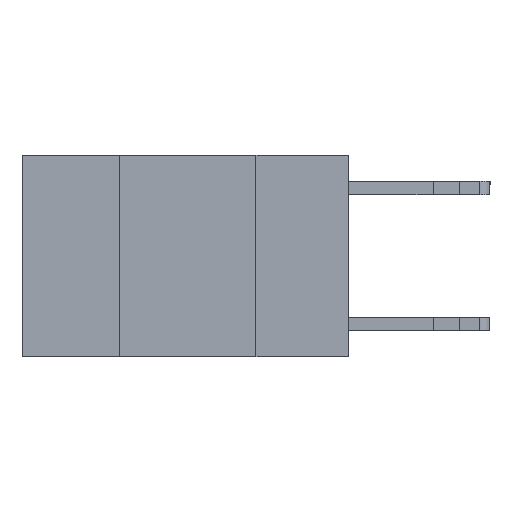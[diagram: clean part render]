
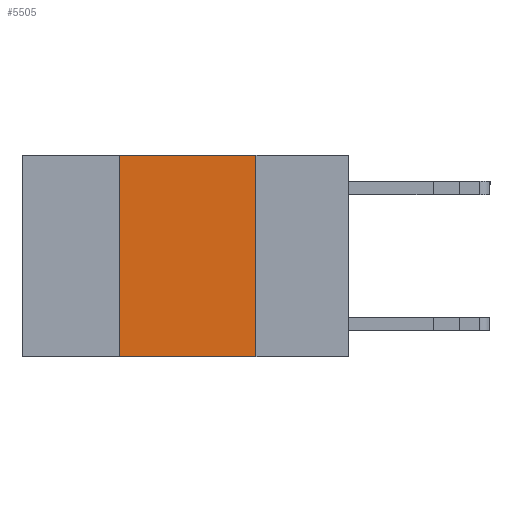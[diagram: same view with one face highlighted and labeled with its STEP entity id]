
A CAD part, left-side view. The second image highlights one B-rep face of the part: STEP entity #5505.
In plain terms, the highlighted planar face has unit normal (-1, 0, 0).
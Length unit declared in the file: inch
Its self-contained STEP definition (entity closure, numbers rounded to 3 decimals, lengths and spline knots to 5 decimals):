
#388 = LINE ( 'NONE', #5888, #15726 ) ;
#2039 = ORIENTED_EDGE ( 'NONE', *, *, #4509, .F. ) ;
#2370 = CARTESIAN_POINT ( 'NONE',  ( 0., 0.42, 0. ) ) ;
#3169 = DIRECTION ( 'NONE',  ( 0., -1., 0. ) ) ;
#3200 = CARTESIAN_POINT ( 'NONE',  ( 0., 0.17, -0.37 ) ) ;
#3448 = VERTEX_POINT ( 'NONE', #3200 ) ;
#3817 = DIRECTION ( 'NONE',  ( 0., 0., 1. ) ) ;
#4509 = EDGE_CURVE ( 'NONE', #7528, #14294, #9182, .T. ) ;
#5053 = ORIENTED_EDGE ( 'NONE', *, *, #5731, .T. ) ;
#5300 = DIRECTION ( 'NONE',  ( 0., 0., -1. ) ) ;
#5437 = VECTOR ( 'NONE', #7919, 39.37008 ) ;
#5505 = ADVANCED_FACE ( 'NONE', ( #9479 ), #9311, .F. ) ;
#5697 = VECTOR ( 'NONE', #11566, 39.37008 ) ;
#5731 = EDGE_CURVE ( 'NONE', #14830, #3448, #388, .T. ) ;
#5888 = CARTESIAN_POINT ( 'NONE',  ( 0., 0.6, -0.37 ) ) ;
#7187 = AXIS2_PLACEMENT_3D ( 'NONE', #17569, #13532, #5300 ) ;
#7528 = VERTEX_POINT ( 'NONE', #15100 ) ;
#7919 = DIRECTION ( 'NONE',  ( 0., 0., -1. ) ) ;
#8011 = CARTESIAN_POINT ( 'NONE',  ( 0., 0.42, -0.37 ) ) ;
#9182 = LINE ( 'NONE', #14190, #5697 ) ;
#9247 = LINE ( 'NONE', #9504, #5437 ) ;
#9311 = PLANE ( 'NONE',  #7187 ) ;
#9479 = FACE_OUTER_BOUND ( 'NONE', #15488, .T. ) ;
#9504 = CARTESIAN_POINT ( 'NONE',  ( 0., 0.17, 0. ) ) ;
#10403 = ORIENTED_EDGE ( 'NONE', *, *, #16967, .F. ) ;
#11566 = DIRECTION ( 'NONE',  ( 0., -1., 0. ) ) ;
#13428 = LINE ( 'NONE', #2370, #15021 ) ;
#13532 = DIRECTION ( 'NONE',  ( 1., 0., 0. ) ) ;
#14190 = CARTESIAN_POINT ( 'NONE',  ( 0., 0.6, 0. ) ) ;
#14294 = VERTEX_POINT ( 'NONE', #14967 ) ;
#14830 = VERTEX_POINT ( 'NONE', #8011 ) ;
#14920 = ORIENTED_EDGE ( 'NONE', *, *, #15795, .F. ) ;
#14967 = CARTESIAN_POINT ( 'NONE',  ( 0., 0.17, 0. ) ) ;
#15021 = VECTOR ( 'NONE', #3817, 39.37008 ) ;
#15100 = CARTESIAN_POINT ( 'NONE',  ( 0., 0.42, 0. ) ) ;
#15488 = EDGE_LOOP ( 'NONE', ( #10403, #2039, #14920, #5053 ) ) ;
#15726 = VECTOR ( 'NONE', #3169, 39.37008 ) ;
#15795 = EDGE_CURVE ( 'NONE', #14830, #7528, #13428, .T. ) ;
#16967 = EDGE_CURVE ( 'NONE', #14294, #3448, #9247, .T. ) ;
#17569 = CARTESIAN_POINT ( 'NONE',  ( 0., 0.6, 0. ) ) ;
